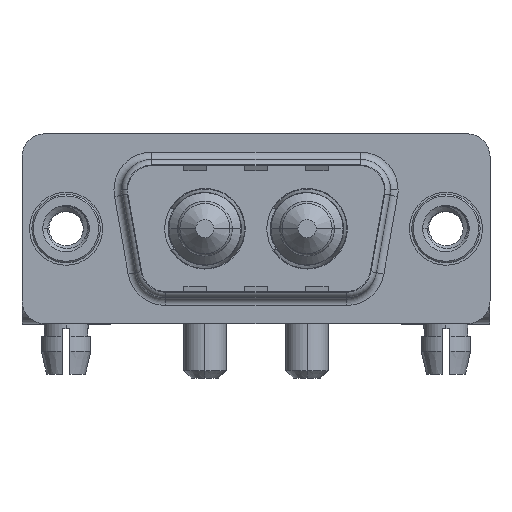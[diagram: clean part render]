
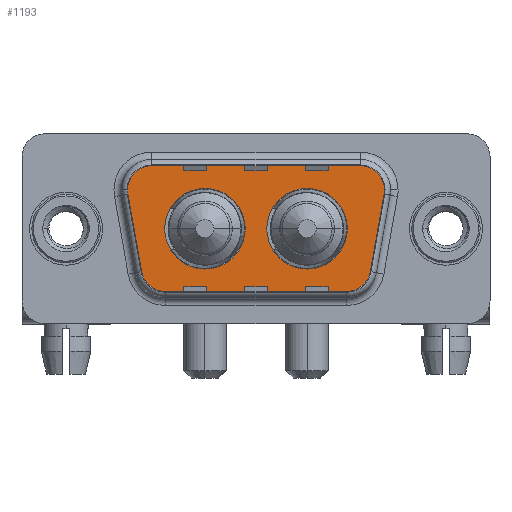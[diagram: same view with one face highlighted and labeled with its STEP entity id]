
A CAD part, top view. The second image highlights one B-rep face of the part: STEP entity #1193.
In plain terms, the highlighted planar face has unit normal (0, 0, 1).
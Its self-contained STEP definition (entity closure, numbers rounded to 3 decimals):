
#117 = DIRECTION ( 'NONE',  ( 1., 0., 0. ) ) ;
#313 = CARTESIAN_POINT ( 'NONE',  ( 6.459, -4.9, 0. ) ) ;
#691 = DIRECTION ( 'NONE',  ( 0., 0., 1. ) ) ;
#700 = VERTEX_POINT ( 'NONE', #7125 ) ;
#712 = CARTESIAN_POINT ( 'NONE',  ( 19.564, 2.9, 0. ) ) ;
#716 = CARTESIAN_POINT ( 'NONE',  ( 5.436, 4.9, 0. ) ) ;
#1172 = DIRECTION ( 'NONE',  ( 0., 0., 1. ) ) ;
#1193 = ADVANCED_FACE ( 'NONE', ( #1241, #3758, #12993 ), #3842, .T. ) ;
#1241 = FACE_BOUND ( 'NONE', #13684, .T. ) ;
#1340 = VERTEX_POINT ( 'NONE', #2988 ) ;
#1430 = EDGE_CURVE ( 'NONE', #7789, #12489, #6429, .T. ) ;
#1447 = CARTESIAN_POINT ( 'NONE',  ( 18.51, 0., 0. ) ) ;
#1660 = CARTESIAN_POINT ( 'NONE',  ( 3.466, 2.553, 0. ) ) ;
#1699 = DIRECTION ( 'NONE',  ( -1., 0., 0. ) ) ;
#1760 = AXIS2_PLACEMENT_3D ( 'NONE', #5674, #10322, #13838 ) ;
#1788 = AXIS2_PLACEMENT_3D ( 'NONE', #4859, #8125, #117 ) ;
#1807 = LINE ( 'NONE', #1660, #11144 ) ;
#2041 = AXIS2_PLACEMENT_3D ( 'NONE', #712, #14746, #14668 ) ;
#2224 = AXIS2_PLACEMENT_3D ( 'NONE', #3224, #10176, #7880 ) ;
#2303 = CARTESIAN_POINT ( 'NONE',  ( 19.564, 4.9, 0. ) ) ;
#2333 = DIRECTION ( 'NONE',  ( 0., 0., 1. ) ) ;
#2574 = EDGE_CURVE ( 'NONE', #5579, #9953, #14002, .T. ) ;
#2804 = EDGE_CURVE ( 'NONE', #5872, #700, #12075, .T. ) ;
#2869 = ORIENTED_EDGE ( 'NONE', *, *, #6828, .F. ) ;
#2896 = DIRECTION ( 'NONE',  ( 1., 0., 0. ) ) ;
#2988 = CARTESIAN_POINT ( 'NONE',  ( 3.466, 2.553, 0. ) ) ;
#3046 = CARTESIAN_POINT ( 'NONE',  ( 6.49, 0., 0. ) ) ;
#3224 = CARTESIAN_POINT ( 'NONE',  ( 5.436, 2.9, 0. ) ) ;
#3439 = EDGE_CURVE ( 'NONE', #9953, #5579, #6940, .T. ) ;
#3510 = DIRECTION ( 'NONE',  ( 0., 0., 1. ) ) ;
#3758 = FACE_BOUND ( 'NONE', #9711, .T. ) ;
#3766 = VECTOR ( 'NONE', #8316, 1000. ) ;
#3818 = CARTESIAN_POINT ( 'NONE',  ( 11.79, 0., 0. ) ) ;
#3842 = PLANE ( 'NONE',  #8389 ) ;
#3854 = DIRECTION ( 'NONE',  ( 1., 0., 0. ) ) ;
#4133 = ORIENTED_EDGE ( 'NONE', *, *, #4791, .T. ) ;
#4434 = EDGE_CURVE ( 'NONE', #4471, #9215, #14789, .T. ) ;
#4471 = VERTEX_POINT ( 'NONE', #9126 ) ;
#4791 = EDGE_CURVE ( 'NONE', #1340, #7257, #1807, .T. ) ;
#4829 = CARTESIAN_POINT ( 'NONE',  ( 9.14, 0., 0. ) ) ;
#4849 = EDGE_LOOP ( 'NONE', ( #6858, #13315, #12292, #13920, #15018, #13117, #4133, #5391, #6634 ) ) ;
#4859 = CARTESIAN_POINT ( 'NONE',  ( 15.86, 0., 0. ) ) ;
#4930 = EDGE_CURVE ( 'NONE', #7257, #5872, #12360, .T. ) ;
#5005 = CARTESIAN_POINT ( 'NONE',  ( 15.86, 0., 0. ) ) ;
#5221 = VERTEX_POINT ( 'NONE', #10160 ) ;
#5391 = ORIENTED_EDGE ( 'NONE', *, *, #4930, .T. ) ;
#5422 = CIRCLE ( 'NONE', #1760, 2. ) ;
#5579 = VERTEX_POINT ( 'NONE', #3046 ) ;
#5674 = CARTESIAN_POINT ( 'NONE',  ( 18.541, -2.9, 0. ) ) ;
#5842 = CARTESIAN_POINT ( 'NONE',  ( 19.564, 2.9, 0. ) ) ;
#5872 = VERTEX_POINT ( 'NONE', #12847 ) ;
#5879 = DIRECTION ( 'NONE',  ( 1., 0., 0. ) ) ;
#5985 = EDGE_CURVE ( 'NONE', #700, #7789, #5422, .T. ) ;
#6164 = VERTEX_POINT ( 'NONE', #10704 ) ;
#6270 = AXIS2_PLACEMENT_3D ( 'NONE', #11687, #10615, #14131 ) ;
#6309 = EDGE_CURVE ( 'NONE', #5221, #1340, #14683, .T. ) ;
#6379 = DIRECTION ( 'NONE',  ( 0.174, -0.985, 0. ) ) ;
#6429 = LINE ( 'NONE', #7427, #13492 ) ;
#6453 = AXIS2_PLACEMENT_3D ( 'NONE', #4829, #3510, #5879 ) ;
#6634 = ORIENTED_EDGE ( 'NONE', *, *, #2804, .T. ) ;
#6828 = EDGE_CURVE ( 'NONE', #6164, #8524, #11746, .T. ) ;
#6858 = ORIENTED_EDGE ( 'NONE', *, *, #5985, .T. ) ;
#6940 = CIRCLE ( 'NONE', #7435, 2.65 ) ;
#7125 = CARTESIAN_POINT ( 'NONE',  ( 18.541, -4.9, 0. ) ) ;
#7194 = DIRECTION ( 'NONE',  ( 1., 0., 0. ) ) ;
#7257 = VERTEX_POINT ( 'NONE', #12335 ) ;
#7427 = CARTESIAN_POINT ( 'NONE',  ( 21.534, 2.553, 0. ) ) ;
#7435 = AXIS2_PLACEMENT_3D ( 'NONE', #10140, #691, #2896 ) ;
#7646 = LINE ( 'NONE', #716, #13790 ) ;
#7789 = VERTEX_POINT ( 'NONE', #10245 ) ;
#7880 = DIRECTION ( 'NONE',  ( 1., 0., 0. ) ) ;
#8125 = DIRECTION ( 'NONE',  ( 0., 0., 1. ) ) ;
#8181 = EDGE_CURVE ( 'NONE', #12489, #4471, #8622, .T. ) ;
#8316 = DIRECTION ( 'NONE',  ( 1., 0., 0. ) ) ;
#8389 = AXIS2_PLACEMENT_3D ( 'NONE', #14215, #1172, #7194 ) ;
#8524 = VERTEX_POINT ( 'NONE', #1447 ) ;
#8622 = CIRCLE ( 'NONE', #2041, 2. ) ;
#9126 = CARTESIAN_POINT ( 'NONE',  ( 21.564, 2.9, 0. ) ) ;
#9215 = VERTEX_POINT ( 'NONE', #2303 ) ;
#9711 = EDGE_LOOP ( 'NONE', ( #11371, #9786 ) ) ;
#9786 = ORIENTED_EDGE ( 'NONE', *, *, #2574, .F. ) ;
#9953 = VERTEX_POINT ( 'NONE', #3818 ) ;
#10140 = CARTESIAN_POINT ( 'NONE',  ( 9.14, 0., 0. ) ) ;
#10160 = CARTESIAN_POINT ( 'NONE',  ( 5.436, 4.9, 0. ) ) ;
#10176 = DIRECTION ( 'NONE',  ( 0., 0., 1. ) ) ;
#10245 = CARTESIAN_POINT ( 'NONE',  ( 20.511, -3.247, 0. ) ) ;
#10322 = DIRECTION ( 'NONE',  ( 0., 0., 1. ) ) ;
#10615 = DIRECTION ( 'NONE',  ( 0., 0., 1. ) ) ;
#10704 = CARTESIAN_POINT ( 'NONE',  ( 13.21, 0., 0. ) ) ;
#11093 = DIRECTION ( 'NONE',  ( 0.174, 0.985, 0. ) ) ;
#11114 = CIRCLE ( 'NONE', #12332, 2.65 ) ;
#11144 = VECTOR ( 'NONE', #6379, 1000. ) ;
#11371 = ORIENTED_EDGE ( 'NONE', *, *, #3439, .F. ) ;
#11494 = DIRECTION ( 'NONE',  ( -1., 0., 0. ) ) ;
#11516 = EDGE_CURVE ( 'NONE', #8524, #6164, #11114, .T. ) ;
#11687 = CARTESIAN_POINT ( 'NONE',  ( 6.459, -2.9, 0. ) ) ;
#11746 = CIRCLE ( 'NONE', #1788, 2.65 ) ;
#11964 = ORIENTED_EDGE ( 'NONE', *, *, #11516, .F. ) ;
#12065 = EDGE_CURVE ( 'NONE', #9215, #5221, #7646, .T. ) ;
#12075 = LINE ( 'NONE', #313, #3766 ) ;
#12292 = ORIENTED_EDGE ( 'NONE', *, *, #8181, .T. ) ;
#12332 = AXIS2_PLACEMENT_3D ( 'NONE', #5005, #14312, #3854 ) ;
#12335 = CARTESIAN_POINT ( 'NONE',  ( 4.489, -3.247, 0. ) ) ;
#12360 = CIRCLE ( 'NONE', #6270, 2. ) ;
#12489 = VERTEX_POINT ( 'NONE', #14504 ) ;
#12847 = CARTESIAN_POINT ( 'NONE',  ( 6.459, -4.9, 0. ) ) ;
#12993 = FACE_OUTER_BOUND ( 'NONE', #4849, .T. ) ;
#13117 = ORIENTED_EDGE ( 'NONE', *, *, #6309, .T. ) ;
#13315 = ORIENTED_EDGE ( 'NONE', *, *, #1430, .T. ) ;
#13492 = VECTOR ( 'NONE', #11093, 1000. ) ;
#13684 = EDGE_LOOP ( 'NONE', ( #11964, #2869 ) ) ;
#13790 = VECTOR ( 'NONE', #1699, 1000. ) ;
#13838 = DIRECTION ( 'NONE',  ( 1., 0., 0. ) ) ;
#13920 = ORIENTED_EDGE ( 'NONE', *, *, #4434, .T. ) ;
#14002 = CIRCLE ( 'NONE', #6453, 2.65 ) ;
#14131 = DIRECTION ( 'NONE',  ( -1., 0., 0. ) ) ;
#14215 = CARTESIAN_POINT ( 'NONE',  ( 18.541, -2.9, 0. ) ) ;
#14312 = DIRECTION ( 'NONE',  ( 0., 0., 1. ) ) ;
#14504 = CARTESIAN_POINT ( 'NONE',  ( 21.534, 2.553, 0. ) ) ;
#14547 = AXIS2_PLACEMENT_3D ( 'NONE', #5842, #2333, #11494 ) ;
#14668 = DIRECTION ( 'NONE',  ( -1., 0., 0. ) ) ;
#14683 = CIRCLE ( 'NONE', #2224, 2. ) ;
#14746 = DIRECTION ( 'NONE',  ( 0., 0., 1. ) ) ;
#14789 = CIRCLE ( 'NONE', #14547, 2. ) ;
#15018 = ORIENTED_EDGE ( 'NONE', *, *, #12065, .T. ) ;
